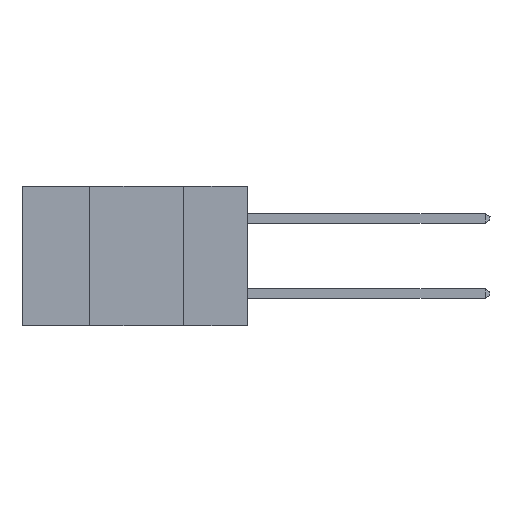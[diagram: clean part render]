
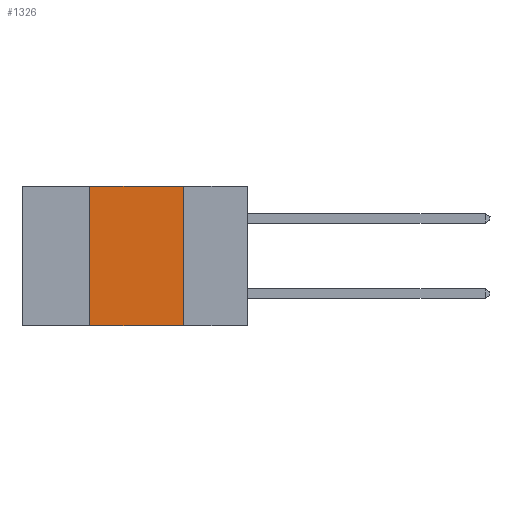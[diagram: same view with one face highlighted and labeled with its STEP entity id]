
A CAD part, left-side view. The second image highlights one B-rep face of the part: STEP entity #1326.
In plain terms, the highlighted planar face has unit normal (-1, 0, 0).
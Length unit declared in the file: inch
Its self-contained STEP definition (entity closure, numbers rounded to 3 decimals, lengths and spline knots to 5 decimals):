
#555 = DIRECTION ( 'NONE',  ( 0., 0., 1. ) ) ;
#831 = VECTOR ( 'NONE', #3730, 39.37008 ) ;
#959 = CARTESIAN_POINT ( 'NONE',  ( 0., 0.42, -0.37 ) ) ;
#1321 = ORIENTED_EDGE ( 'NONE', *, *, #3225, .F. ) ;
#1326 = ADVANCED_FACE ( 'NONE', ( #8605 ), #12431, .F. ) ;
#1568 = EDGE_CURVE ( 'NONE', #8490, #1831, #5936, .T. ) ;
#1831 = VERTEX_POINT ( 'NONE', #7889 ) ;
#2587 = VERTEX_POINT ( 'NONE', #959 ) ;
#3225 = EDGE_CURVE ( 'NONE', #11139, #8490, #4368, .T. ) ;
#3529 = ORIENTED_EDGE ( 'NONE', *, *, #12266, .F. ) ;
#3535 = EDGE_CURVE ( 'NONE', #2587, #1831, #4737, .T. ) ;
#3660 = ORIENTED_EDGE ( 'NONE', *, *, #3535, .T. ) ;
#3730 = DIRECTION ( 'NONE',  ( 0., -1., 0. ) ) ;
#3827 = CARTESIAN_POINT ( 'NONE',  ( 0., 0.6, 0. ) ) ;
#4066 = CARTESIAN_POINT ( 'NONE',  ( 0., 0.42, 0. ) ) ;
#4368 = LINE ( 'NONE', #6293, #6441 ) ;
#4737 = LINE ( 'NONE', #4794, #831 ) ;
#4794 = CARTESIAN_POINT ( 'NONE',  ( 0., 0.6, -0.37 ) ) ;
#5003 = CARTESIAN_POINT ( 'NONE',  ( 0., 0.17, -0.37 ) ) ;
#5096 = VECTOR ( 'NONE', #555, 39.37008 ) ;
#5140 = ORIENTED_EDGE ( 'NONE', *, *, #1568, .F. ) ;
#5755 = DIRECTION ( 'NONE',  ( 0., 0., -1. ) ) ;
#5936 = LINE ( 'NONE', #5003, #9415 ) ;
#6171 = DIRECTION ( 'NONE',  ( 0., -1., 0. ) ) ;
#6293 = CARTESIAN_POINT ( 'NONE',  ( 0., 0.6, 0. ) ) ;
#6441 = VECTOR ( 'NONE', #6171, 39.37008 ) ;
#7247 = EDGE_LOOP ( 'NONE', ( #5140, #1321, #3529, #3660 ) ) ;
#7647 = DIRECTION ( 'NONE',  ( 1., 0., 0. ) ) ;
#7889 = CARTESIAN_POINT ( 'NONE',  ( 0., 0.17, -0.37 ) ) ;
#8234 = LINE ( 'NONE', #10128, #5096 ) ;
#8490 = VERTEX_POINT ( 'NONE', #9999 ) ;
#8605 = FACE_OUTER_BOUND ( 'NONE', #7247, .T. ) ;
#9415 = VECTOR ( 'NONE', #10475, 39.37008 ) ;
#9999 = CARTESIAN_POINT ( 'NONE',  ( 0., 0.17, 0. ) ) ;
#10128 = CARTESIAN_POINT ( 'NONE',  ( 0., 0.42, -0.37 ) ) ;
#10475 = DIRECTION ( 'NONE',  ( 0., 0., -1. ) ) ;
#10854 = AXIS2_PLACEMENT_3D ( 'NONE', #3827, #7647, #5755 ) ;
#11139 = VERTEX_POINT ( 'NONE', #4066 ) ;
#12266 = EDGE_CURVE ( 'NONE', #2587, #11139, #8234, .T. ) ;
#12431 = PLANE ( 'NONE',  #10854 ) ;
